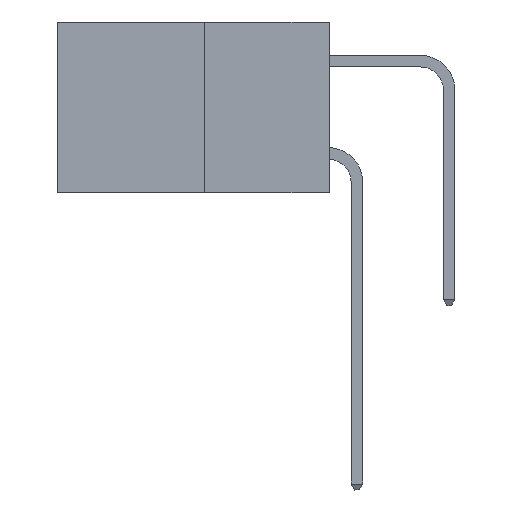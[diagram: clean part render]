
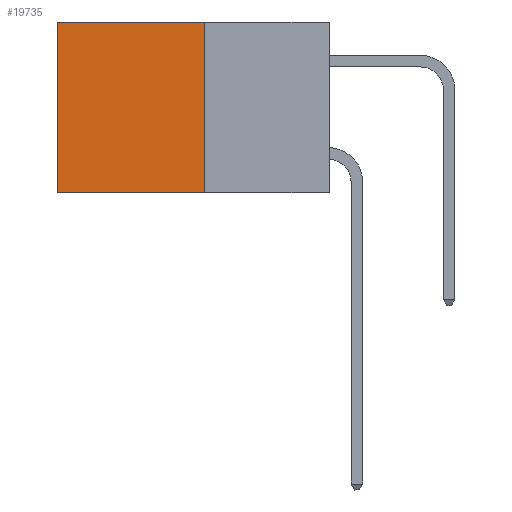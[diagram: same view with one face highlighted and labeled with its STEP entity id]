
A CAD part, left-side view. The second image highlights one B-rep face of the part: STEP entity #19735.
In plain terms, the highlighted planar face has unit normal (-1, 0, 0).
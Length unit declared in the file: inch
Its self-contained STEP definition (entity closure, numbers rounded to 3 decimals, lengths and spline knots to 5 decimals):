
#1158 = ORIENTED_EDGE ( 'NONE', *, *, #14119, .T. ) ;
#1367 = CARTESIAN_POINT ( 'NONE',  ( 0.277, 0.27, 0. ) ) ;
#1576 = CARTESIAN_POINT ( 'NONE',  ( 0.277, 0.27, 0. ) ) ;
#1604 = VERTEX_POINT ( 'NONE', #19955 ) ;
#2888 = CARTESIAN_POINT ( 'NONE',  ( 0.277, 0.27, -0.37 ) ) ;
#3308 = VERTEX_POINT ( 'NONE', #1367 ) ;
#3543 = VERTEX_POINT ( 'NONE', #17646 ) ;
#4150 = PLANE ( 'NONE',  #21847 ) ;
#5885 = CARTESIAN_POINT ( 'NONE',  ( 0.277, 0.27, -0.37 ) ) ;
#7753 = DIRECTION ( 'NONE',  ( 1., 0., 0. ) ) ;
#9352 = EDGE_LOOP ( 'NONE', ( #1158, #16554, #12067, #14292 ) ) ;
#10069 = DIRECTION ( 'NONE',  ( 0., 0., -1. ) ) ;
#10456 = EDGE_CURVE ( 'NONE', #3308, #3543, #20882, .T. ) ;
#11134 = VECTOR ( 'NONE', #13998, 39.37008 ) ;
#12067 = ORIENTED_EDGE ( 'NONE', *, *, #21267, .F. ) ;
#13224 = VECTOR ( 'NONE', #10069, 39.37008 ) ;
#13998 = DIRECTION ( 'NONE',  ( 0., 1., 0. ) ) ;
#14119 = EDGE_CURVE ( 'NONE', #3543, #1604, #16686, .T. ) ;
#14292 = ORIENTED_EDGE ( 'NONE', *, *, #10456, .T. ) ;
#14825 = DIRECTION ( 'NONE',  ( 0., 1., 0. ) ) ;
#15998 = VECTOR ( 'NONE', #14825, 39.37008 ) ;
#16042 = CARTESIAN_POINT ( 'NONE',  ( 0.277, 0.59, -0.37 ) ) ;
#16507 = FACE_OUTER_BOUND ( 'NONE', #9352, .T. ) ;
#16554 = ORIENTED_EDGE ( 'NONE', *, *, #21081, .F. ) ;
#16686 = LINE ( 'NONE', #16042, #20698 ) ;
#17549 = CARTESIAN_POINT ( 'NONE',  ( 0.277, 0.27, -0.37 ) ) ;
#17646 = CARTESIAN_POINT ( 'NONE',  ( 0.277, 0.59, 0. ) ) ;
#17764 = DIRECTION ( 'NONE',  ( 0., 0., -1. ) ) ;
#19524 = VERTEX_POINT ( 'NONE', #17549 ) ;
#19735 = ADVANCED_FACE ( 'NONE', ( #16507 ), #4150, .F. ) ;
#19928 = DIRECTION ( 'NONE',  ( 0., 0., -1. ) ) ;
#19955 = CARTESIAN_POINT ( 'NONE',  ( 0.277, 0.59, -0.37 ) ) ;
#20544 = LINE ( 'NONE', #21634, #15998 ) ;
#20698 = VECTOR ( 'NONE', #17764, 39.37008 ) ;
#20882 = LINE ( 'NONE', #1576, #11134 ) ;
#21081 = EDGE_CURVE ( 'NONE', #19524, #1604, #20544, .T. ) ;
#21267 = EDGE_CURVE ( 'NONE', #3308, #19524, #21845, .T. ) ;
#21634 = CARTESIAN_POINT ( 'NONE',  ( 0.277, 0.27, -0.37 ) ) ;
#21845 = LINE ( 'NONE', #2888, #13224 ) ;
#21847 = AXIS2_PLACEMENT_3D ( 'NONE', #5885, #7753, #19928 ) ;
